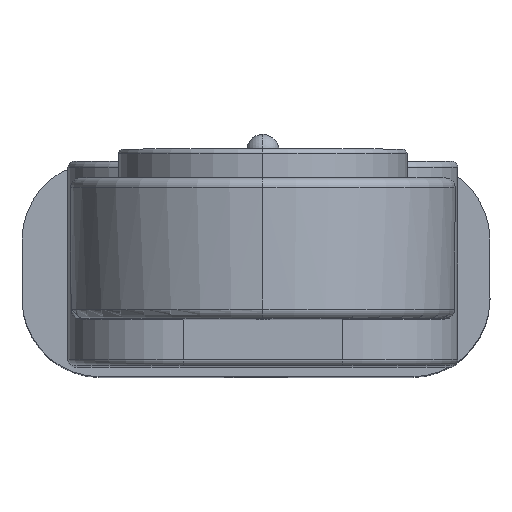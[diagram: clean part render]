
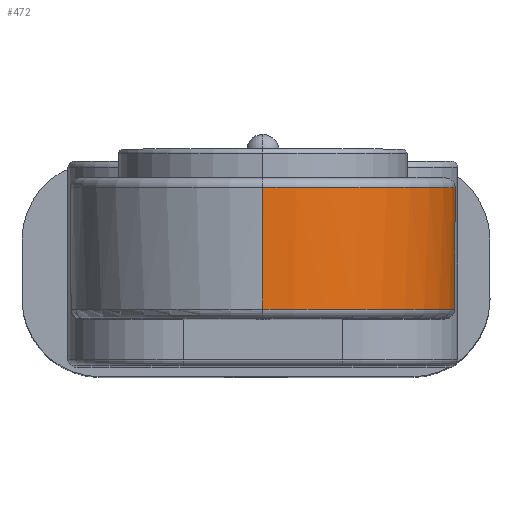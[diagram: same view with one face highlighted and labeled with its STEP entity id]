
A CAD part, top view. The second image highlights one B-rep face of the part: STEP entity #472.
In plain terms, the highlighted cylindrical face has radius 6 mm (diameter 12 mm), a partial arc.
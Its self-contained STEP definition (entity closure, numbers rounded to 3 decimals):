
#114 = DIRECTION ( 'NONE',  ( 0., 0., 1. ) ) ;
#135 = EDGE_CURVE ( 'NONE', #5721, #589, #3508, .T. ) ;
#333 = CARTESIAN_POINT ( 'NONE',  ( 2.5, 3.7, -5.454 ) ) ;
#352 = LINE ( 'NONE', #6377, #5984 ) ;
#373 = B_SPLINE_CURVE_WITH_KNOTS ( 'NONE', 3,
 ( #1346, #2316, #5936, #5867, #797, #333 ),
 .UNSPECIFIED., .F., .F.,
 ( 4, 2, 4 ),
 ( 0., 0., 0. ),
 .UNSPECIFIED. ) ;
#452 = CIRCLE ( 'NONE', #1175, 6. ) ;
#472 = ADVANCED_FACE ( 'NONE', ( #3006 ), #4504, .T. ) ;
#589 = VERTEX_POINT ( 'NONE', #4159 ) ;
#597 = CARTESIAN_POINT ( 'NONE',  ( 2.8, 4.4, -5.307 ) ) ;
#634 = EDGE_CURVE ( 'NONE', #5742, #5721, #2059, .T. ) ;
#794 = EDGE_CURVE ( 'NONE', #5493, #5742, #352, .T. ) ;
#797 = CARTESIAN_POINT ( 'NONE',  ( 2.576, 3.7, -5.42 ) ) ;
#877 = AXIS2_PLACEMENT_3D ( 'NONE', #3715, #5745, #114 ) ;
#910 = EDGE_CURVE ( 'NONE', #2131, #3559, #4492, .T. ) ;
#1175 = AXIS2_PLACEMENT_3D ( 'NONE', #3843, #2317, #1879 ) ;
#1270 = ORIENTED_EDGE ( 'NONE', *, *, #135, .T. ) ;
#1284 = ORIENTED_EDGE ( 'NONE', *, *, #6408, .T. ) ;
#1301 = ORIENTED_EDGE ( 'NONE', *, *, #910, .F. ) ;
#1346 = CARTESIAN_POINT ( 'NONE',  ( 2.8, 3.4, -5.307 ) ) ;
#1555 = EDGE_LOOP ( 'NONE', ( #2902, #5112, #1970, #1270, #1284, #4777, #1301 ) ) ;
#1699 = DIRECTION ( 'NONE',  ( 0., 0., 1. ) ) ;
#1879 = DIRECTION ( 'NONE',  ( 0., 0., 1. ) ) ;
#1970 = ORIENTED_EDGE ( 'NONE', *, *, #634, .T. ) ;
#2059 = CIRCLE ( 'NONE', #5868, 6. ) ;
#2131 = VERTEX_POINT ( 'NONE', #3114 ) ;
#2172 = AXIS2_PLACEMENT_3D ( 'NONE', #3037, #3070, #6148 ) ;
#2254 = CARTESIAN_POINT ( 'NONE',  ( 0., 3.7, -6. ) ) ;
#2316 = CARTESIAN_POINT ( 'NONE',  ( 2.8, 3.484, -5.307 ) ) ;
#2317 = DIRECTION ( 'NONE',  ( 0., 1., 0. ) ) ;
#2811 = VECTOR ( 'NONE', #3060, 1000. ) ;
#2902 = ORIENTED_EDGE ( 'NONE', *, *, #3103, .T. ) ;
#2920 = CARTESIAN_POINT ( 'NONE',  ( 2.8, 0.3, -5.307 ) ) ;
#3006 = FACE_OUTER_BOUND ( 'NONE', #1555, .T. ) ;
#3037 = CARTESIAN_POINT ( 'NONE',  ( 0., 4.4, 0. ) ) ;
#3060 = DIRECTION ( 'NONE',  ( 0., -1., 0. ) ) ;
#3070 = DIRECTION ( 'NONE',  ( 0., -1., 0. ) ) ;
#3089 = CARTESIAN_POINT ( 'NONE',  ( 0., 4.1, 6. ) ) ;
#3103 = EDGE_CURVE ( 'NONE', #2131, #5493, #3724, .T. ) ;
#3114 = CARTESIAN_POINT ( 'NONE',  ( 0., 4.1, -6. ) ) ;
#3508 = LINE ( 'NONE', #597, #4521 ) ;
#3559 = VERTEX_POINT ( 'NONE', #2254 ) ;
#3715 = CARTESIAN_POINT ( 'NONE',  ( 0., 4.1, 0. ) ) ;
#3724 = CIRCLE ( 'NONE', #877, 6. ) ;
#3843 = CARTESIAN_POINT ( 'NONE',  ( 0., 3.7, 0. ) ) ;
#3940 = CARTESIAN_POINT ( 'NONE',  ( 0., 0.3, 6. ) ) ;
#4159 = CARTESIAN_POINT ( 'NONE',  ( 2.8, 3.4, -5.307 ) ) ;
#4492 = LINE ( 'NONE', #6017, #2811 ) ;
#4504 = CYLINDRICAL_SURFACE ( 'NONE', #2172, 6. ) ;
#4521 = VECTOR ( 'NONE', #5658, 1000. ) ;
#4690 = CARTESIAN_POINT ( 'NONE',  ( 0., 0.3, 0. ) ) ;
#4777 = ORIENTED_EDGE ( 'NONE', *, *, #5724, .T. ) ;
#5112 = ORIENTED_EDGE ( 'NONE', *, *, #794, .T. ) ;
#5493 = VERTEX_POINT ( 'NONE', #3089 ) ;
#5658 = DIRECTION ( 'NONE',  ( 0., 1., 0. ) ) ;
#5721 = VERTEX_POINT ( 'NONE', #2920 ) ;
#5724 = EDGE_CURVE ( 'NONE', #5732, #3559, #452, .T. ) ;
#5732 = VERTEX_POINT ( 'NONE', #5869 ) ;
#5742 = VERTEX_POINT ( 'NONE', #3940 ) ;
#5745 = DIRECTION ( 'NONE',  ( 0., -1., 0. ) ) ;
#5867 = CARTESIAN_POINT ( 'NONE',  ( 2.65, 3.671, -5.383 ) ) ;
#5868 = AXIS2_PLACEMENT_3D ( 'NONE', #4690, #6245, #1699 ) ;
#5869 = CARTESIAN_POINT ( 'NONE',  ( 2.5, 3.7, -5.454 ) ) ;
#5936 = CARTESIAN_POINT ( 'NONE',  ( 2.763, 3.564, -5.326 ) ) ;
#5984 = VECTOR ( 'NONE', #6406, 1000. ) ;
#6017 = CARTESIAN_POINT ( 'NONE',  ( 0., 4.4, -6. ) ) ;
#6148 = DIRECTION ( 'NONE',  ( 0., 0., -1. ) ) ;
#6245 = DIRECTION ( 'NONE',  ( 0., 1., 0. ) ) ;
#6377 = CARTESIAN_POINT ( 'NONE',  ( 0., 4.4, 6. ) ) ;
#6406 = DIRECTION ( 'NONE',  ( 0., -1., 0. ) ) ;
#6408 = EDGE_CURVE ( 'NONE', #589, #5732, #373, .T. ) ;
